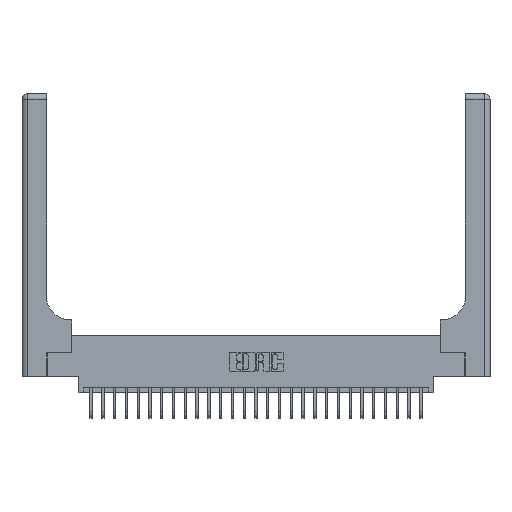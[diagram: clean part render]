
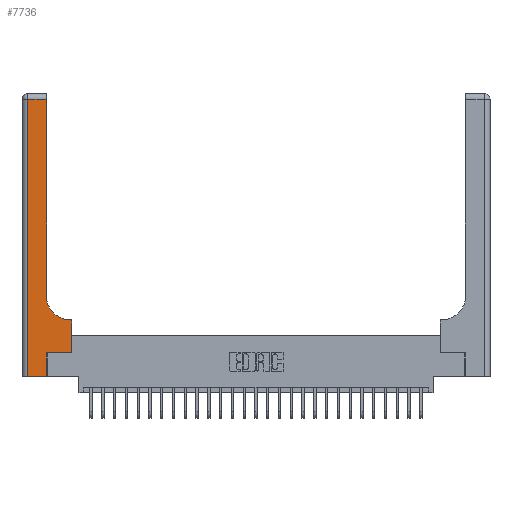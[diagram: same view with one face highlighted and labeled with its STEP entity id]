
A CAD part, top view. The second image highlights one B-rep face of the part: STEP entity #7736.
In plain terms, the highlighted planar face has unit normal (0, 0, 1).
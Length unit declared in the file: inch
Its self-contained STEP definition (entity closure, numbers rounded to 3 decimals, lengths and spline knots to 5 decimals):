
#567 = EDGE_CURVE ( 'NONE', #23895, #12793, #2003, .T. ) ;
#585 = CARTESIAN_POINT ( 'NONE',  ( 0.26, 2.94, 0.37 ) ) ;
#973 = VECTOR ( 'NONE', #21064, 39.37008 ) ;
#1066 = CARTESIAN_POINT ( 'NONE',  ( 0.265, 0., 0.37 ) ) ;
#1133 = CARTESIAN_POINT ( 'NONE',  ( 0.528, 0.6, 0.37 ) ) ;
#1460 = LINE ( 'NONE', #20742, #20591 ) ;
#1517 = CARTESIAN_POINT ( 'NONE',  ( 0., 0., 0.37 ) ) ;
#1551 = EDGE_CURVE ( 'NONE', #16907, #11728, #25319, .T. ) ;
#1730 = ORIENTED_EDGE ( 'NONE', *, *, #567, .T. ) ;
#2003 = LINE ( 'NONE', #19490, #21723 ) ;
#2138 = ORIENTED_EDGE ( 'NONE', *, *, #21267, .T. ) ;
#2217 = DIRECTION ( 'NONE',  ( 0., 1., 0. ) ) ;
#2267 = VECTOR ( 'NONE', #2217, 39.37008 ) ;
#2284 = DIRECTION ( 'NONE',  ( -1., 0., 0. ) ) ;
#3011 = DIRECTION ( 'NONE',  ( -1., 0., 0. ) ) ;
#3625 = ORIENTED_EDGE ( 'NONE', *, *, #4504, .T. ) ;
#3915 = CARTESIAN_POINT ( 'NONE',  ( 0.51, 0.85, 0.37 ) ) ;
#4156 = LINE ( 'NONE', #13757, #2267 ) ;
#4412 = VERTEX_POINT ( 'NONE', #10001 ) ;
#4504 = EDGE_CURVE ( 'NONE', #23079, #14744, #10513, .T. ) ;
#4688 = VERTEX_POINT ( 'NONE', #23187 ) ;
#4927 = AXIS2_PLACEMENT_3D ( 'NONE', #8119, #17710, #2284 ) ;
#5246 = ORIENTED_EDGE ( 'NONE', *, *, #18297, .T. ) ;
#5612 = DIRECTION ( 'NONE',  ( 1., 0., 0. ) ) ;
#5951 = EDGE_CURVE ( 'NONE', #12793, #4688, #1460, .T. ) ;
#6330 = VECTOR ( 'NONE', #19627, 39.37008 ) ;
#7457 = LINE ( 'NONE', #9907, #6330 ) ;
#7725 = ORIENTED_EDGE ( 'NONE', *, *, #22173, .T. ) ;
#7736 = ADVANCED_FACE ( 'NONE', ( #9932 ), #18080, .F. ) ;
#8119 = CARTESIAN_POINT ( 'NONE',  ( 0., 3., 0.37 ) ) ;
#8671 = EDGE_CURVE ( 'NONE', #4688, #4412, #12603, .T. ) ;
#8992 = CARTESIAN_POINT ( 'NONE',  ( 0.528, 0.25, 0.37 ) ) ;
#9717 = LINE ( 'NONE', #17368, #18657 ) ;
#9736 = ORIENTED_EDGE ( 'NONE', *, *, #13068, .T. ) ;
#9872 = DIRECTION ( 'NONE',  ( 0., 0., -1. ) ) ;
#9907 = CARTESIAN_POINT ( 'NONE',  ( 0.26, 3., 0.37 ) ) ;
#9932 = FACE_OUTER_BOUND ( 'NONE', #19646, .T. ) ;
#10001 = CARTESIAN_POINT ( 'NONE',  ( 0.26, 0.85, 0.37 ) ) ;
#10260 = CARTESIAN_POINT ( 'NONE',  ( 0., 2.94, 0.37 ) ) ;
#10363 = DIRECTION ( 'NONE',  ( 0., -1., 0. ) ) ;
#10513 = LINE ( 'NONE', #10260, #12050 ) ;
#10529 = AXIS2_PLACEMENT_3D ( 'NONE', #3915, #9872, #5612 ) ;
#11728 = VERTEX_POINT ( 'NONE', #1066 ) ;
#12050 = VECTOR ( 'NONE', #14677, 39.37008 ) ;
#12090 = DIRECTION ( 'NONE',  ( 0., 1., 0. ) ) ;
#12315 = LINE ( 'NONE', #20208, #20857 ) ;
#12603 = CIRCLE ( 'NONE', #10529, 0.25 ) ;
#12793 = VERTEX_POINT ( 'NONE', #1133 ) ;
#13068 = EDGE_CURVE ( 'NONE', #21018, #23895, #9717, .T. ) ;
#13757 = CARTESIAN_POINT ( 'NONE',  ( 0.265, 0., 0.37 ) ) ;
#14677 = DIRECTION ( 'NONE',  ( -1., 0., 0. ) ) ;
#14744 = VERTEX_POINT ( 'NONE', #16879 ) ;
#16879 = CARTESIAN_POINT ( 'NONE',  ( 0.06, 2.94, 0.37 ) ) ;
#16907 = VERTEX_POINT ( 'NONE', #23336 ) ;
#17368 = CARTESIAN_POINT ( 'NONE',  ( 0.265, 0.25, 0.37 ) ) ;
#17710 = DIRECTION ( 'NONE',  ( 0., 0., -1. ) ) ;
#17879 = CARTESIAN_POINT ( 'NONE',  ( 0.265, 0.25, 0.37 ) ) ;
#17934 = ORIENTED_EDGE ( 'NONE', *, *, #8671, .T. ) ;
#18080 = PLANE ( 'NONE',  #4927 ) ;
#18297 = EDGE_CURVE ( 'NONE', #4412, #23079, #7457, .T. ) ;
#18657 = VECTOR ( 'NONE', #25254, 39.37008 ) ;
#19490 = CARTESIAN_POINT ( 'NONE',  ( 0.528, 0.25, 0.37 ) ) ;
#19627 = DIRECTION ( 'NONE',  ( 0., 1., 0. ) ) ;
#19646 = EDGE_LOOP ( 'NONE', ( #5246, #3625, #2138, #22544, #7725, #9736, #1730, #23057, #17934 ) ) ;
#20208 = CARTESIAN_POINT ( 'NONE',  ( 0.06, 3., 0.37 ) ) ;
#20591 = VECTOR ( 'NONE', #3011, 39.37008 ) ;
#20742 = CARTESIAN_POINT ( 'NONE',  ( 0.26, 0.6, 0.37 ) ) ;
#20857 = VECTOR ( 'NONE', #10363, 39.37008 ) ;
#21018 = VERTEX_POINT ( 'NONE', #17879 ) ;
#21064 = DIRECTION ( 'NONE',  ( 1., 0., 0. ) ) ;
#21267 = EDGE_CURVE ( 'NONE', #14744, #16907, #12315, .T. ) ;
#21723 = VECTOR ( 'NONE', #12090, 39.37008 ) ;
#22173 = EDGE_CURVE ( 'NONE', #11728, #21018, #4156, .T. ) ;
#22544 = ORIENTED_EDGE ( 'NONE', *, *, #1551, .T. ) ;
#23057 = ORIENTED_EDGE ( 'NONE', *, *, #5951, .T. ) ;
#23079 = VERTEX_POINT ( 'NONE', #585 ) ;
#23187 = CARTESIAN_POINT ( 'NONE',  ( 0.51, 0.6, 0.37 ) ) ;
#23336 = CARTESIAN_POINT ( 'NONE',  ( 0.06, 0., 0.37 ) ) ;
#23895 = VERTEX_POINT ( 'NONE', #8992 ) ;
#25254 = DIRECTION ( 'NONE',  ( 1., 0., 0. ) ) ;
#25319 = LINE ( 'NONE', #1517, #973 ) ;
